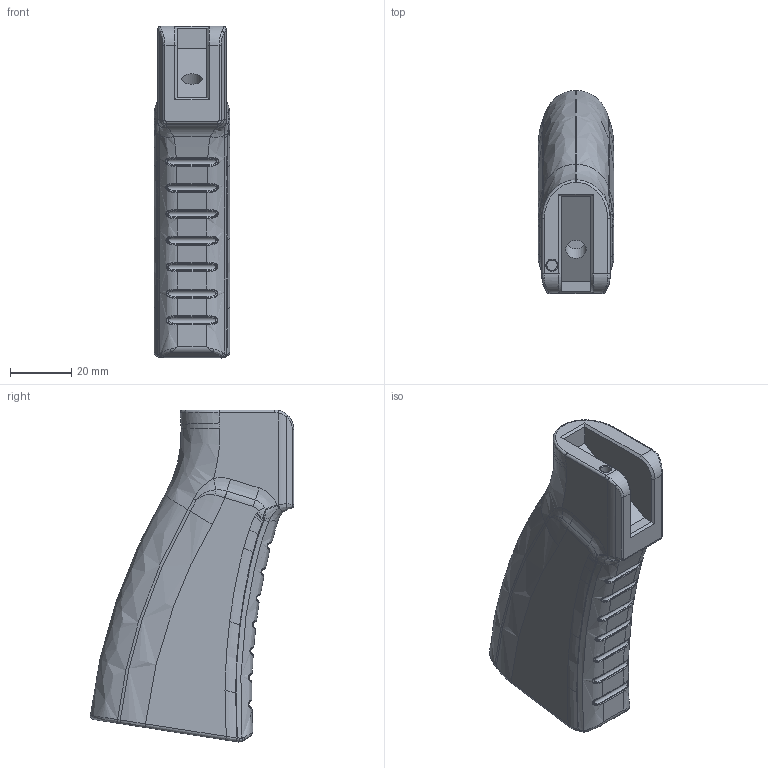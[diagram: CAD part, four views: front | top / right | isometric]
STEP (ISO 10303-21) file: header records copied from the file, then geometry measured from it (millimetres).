
FILE_DESCRIPTION(/* description */ (''),/* implementation_level */ '2;1');
FILE_NAME(/* name */ 'Ridged.step',/* time_stamp */ '2021-07-06T20:45:04-04:00',/* author */ (''),/* organization */ (''),/* preprocessor_version */ 'ST-DEVELOPER v18.1',/* originating_system */ 'Autodesk Translation Framework v10.9.0.1377',/* authorisation */ '');
FILE_SCHEMA (('AUTOMOTIVE_DESIGN { 1 0 10303 214 3 1 1 }'));
Length unit declared in the file: millimetre
Products named in the file (1): Ridged
Bounding box: 24.83 x 66.65 x 108.78 mm (x, y, z)
Volume: 57041.1 mm3; surface area: 23379.4 mm2
Topology: 1 solids, 1 shells, 409 faces, 979 edges, 561 vertices
Faces by surface type: bspline 232, cylinder 87, plane 50, torus 35, cone 5
Full cylindrical faces by diameter (mm): 3.4 x1, 6.8 x1, 11.05 x1, 12.75 x1
Entity records: 20147 total; most frequent: CARTESIAN_POINT 12126, ORIENTED_EDGE 1922, DIRECTION 1216, EDGE_CURVE 961, VERTEX_POINT 561, AXIS2_PLACEMENT_3D 502, B_SPLINE_CURVE_WITH_KNOTS 425, EDGE_LOOP 418
